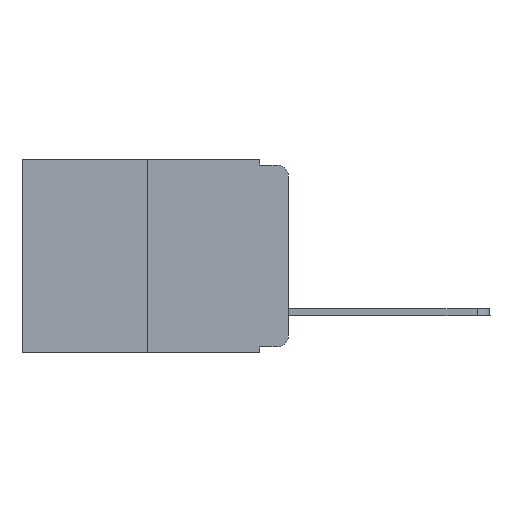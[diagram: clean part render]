
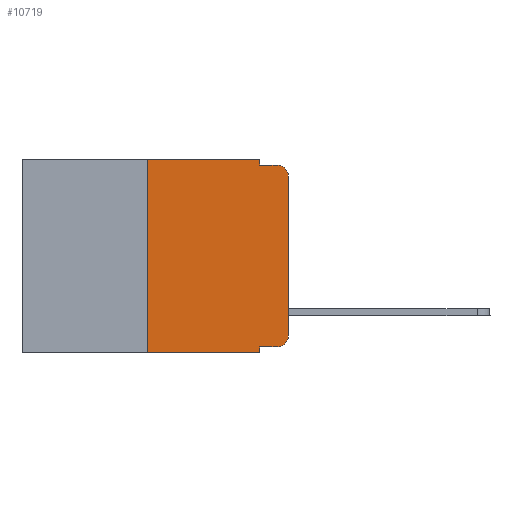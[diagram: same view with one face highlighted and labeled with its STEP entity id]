
A CAD part, left-side view. The second image highlights one B-rep face of the part: STEP entity #10719.
In plain terms, the highlighted planar face has unit normal (-1, 0, 0).
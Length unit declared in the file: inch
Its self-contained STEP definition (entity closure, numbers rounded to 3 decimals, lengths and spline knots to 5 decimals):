
#360 = CARTESIAN_POINT ( 'NONE',  ( 0., 0.051, -0.01 ) ) ;
#412 = VERTEX_POINT ( 'NONE', #360 ) ;
#806 = EDGE_CURVE ( 'NONE', #16024, #5300, #3020, .T. ) ;
#1102 = AXIS2_PLACEMENT_3D ( 'NONE', #13139, #18219, #8176 ) ;
#1482 = CARTESIAN_POINT ( 'NONE',  ( 0., 0.25, -0.343 ) ) ;
#1589 = DIRECTION ( 'NONE',  ( 0., 0., 1. ) ) ;
#2037 = DIRECTION ( 'NONE',  ( -1., 0., 0. ) ) ;
#2139 = CARTESIAN_POINT ( 'NONE',  ( 0., 0.051, -0.343 ) ) ;
#2553 = AXIS2_PLACEMENT_3D ( 'NONE', #12079, #2037, #7102 ) ;
#3020 = LINE ( 'NONE', #21550, #20329 ) ;
#3321 = VECTOR ( 'NONE', #19621, 39.37008 ) ;
#3622 = EDGE_CURVE ( 'NONE', #412, #6630, #21020, .T. ) ;
#3847 = ORIENTED_EDGE ( 'NONE', *, *, #3622, .F. ) ;
#4429 = LINE ( 'NONE', #4754, #17223 ) ;
#4602 = VECTOR ( 'NONE', #11974, 39.37008 ) ;
#4754 = CARTESIAN_POINT ( 'NONE',  ( 0., 0.473, -0.343 ) ) ;
#4831 = ORIENTED_EDGE ( 'NONE', *, *, #13532, .T. ) ;
#4868 = DIRECTION ( 'NONE',  ( 0., 0., -1. ) ) ;
#5271 = VECTOR ( 'NONE', #1589, 39.37008 ) ;
#5300 = VERTEX_POINT ( 'NONE', #2139 ) ;
#5643 = ORIENTED_EDGE ( 'NONE', *, *, #19200, .T. ) ;
#5779 = EDGE_CURVE ( 'NONE', #13026, #412, #11956, .T. ) ;
#5820 = VERTEX_POINT ( 'NONE', #17259 ) ;
#5857 = CARTESIAN_POINT ( 'NONE',  ( 0., 0.02, -0.333 ) ) ;
#5934 = DIRECTION ( 'NONE',  ( 0., -1., 0. ) ) ;
#6144 = VECTOR ( 'NONE', #17439, 39.37008 ) ;
#6237 = CARTESIAN_POINT ( 'NONE',  ( 0., 0.25, 0. ) ) ;
#6418 = CARTESIAN_POINT ( 'NONE',  ( 0., 0., -0.313 ) ) ;
#6488 = ORIENTED_EDGE ( 'NONE', *, *, #5779, .F. ) ;
#6512 = DIRECTION ( 'NONE',  ( 0., 0., -1. ) ) ;
#6630 = VERTEX_POINT ( 'NONE', #7505 ) ;
#7102 = DIRECTION ( 'NONE',  ( 0., 0., -1. ) ) ;
#7472 = EDGE_CURVE ( 'NONE', #21253, #19652, #8173, .T. ) ;
#7505 = CARTESIAN_POINT ( 'NONE',  ( 0., 0.02, -0.01 ) ) ;
#8173 = LINE ( 'NONE', #19317, #5271 ) ;
#8176 = DIRECTION ( 'NONE',  ( 0., 0., -1. ) ) ;
#9344 = EDGE_LOOP ( 'NONE', ( #11230, #16043, #3847, #6488, #15155, #11465, #5643, #19975, #10318, #4831 ) ) ;
#9807 = CIRCLE ( 'NONE', #2553, 0.02 ) ;
#9968 = EDGE_CURVE ( 'NONE', #19652, #13026, #12210, .T. ) ;
#10035 = DIRECTION ( 'NONE',  ( 1., 0., 0. ) ) ;
#10048 = LINE ( 'NONE', #17512, #6144 ) ;
#10067 = EDGE_CURVE ( 'NONE', #5820, #6630, #17485, .T. ) ;
#10318 = ORIENTED_EDGE ( 'NONE', *, *, #12422, .T. ) ;
#10517 = CARTESIAN_POINT ( 'NONE',  ( 0., 0.051, 0. ) ) ;
#10578 = LINE ( 'NONE', #13588, #4602 ) ;
#10644 = CARTESIAN_POINT ( 'NONE',  ( 0., 0.051, 0. ) ) ;
#10719 = ADVANCED_FACE ( 'NONE', ( #13483 ), #16716, .F. ) ;
#11230 = ORIENTED_EDGE ( 'NONE', *, *, #11560, .T. ) ;
#11465 = ORIENTED_EDGE ( 'NONE', *, *, #7472, .F. ) ;
#11560 = EDGE_CURVE ( 'NONE', #17374, #5820, #10048, .T. ) ;
#11956 = LINE ( 'NONE', #10517, #16962 ) ;
#11974 = DIRECTION ( 'NONE',  ( 0., -1., 0. ) ) ;
#12079 = CARTESIAN_POINT ( 'NONE',  ( 0., 0.02, -0.313 ) ) ;
#12210 = LINE ( 'NONE', #14386, #3321 ) ;
#12353 = CARTESIAN_POINT ( 'NONE',  ( 0., 0.051, -0.01 ) ) ;
#12422 = EDGE_CURVE ( 'NONE', #16024, #12492, #10578, .T. ) ;
#12492 = VERTEX_POINT ( 'NONE', #5857 ) ;
#13026 = VERTEX_POINT ( 'NONE', #10644 ) ;
#13139 = CARTESIAN_POINT ( 'NONE',  ( 0., 0.02, -0.03 ) ) ;
#13483 = FACE_OUTER_BOUND ( 'NONE', #9344, .T. ) ;
#13532 = EDGE_CURVE ( 'NONE', #12492, #17374, #9807, .T. ) ;
#13588 = CARTESIAN_POINT ( 'NONE',  ( 0., 0.051, -0.333 ) ) ;
#14386 = CARTESIAN_POINT ( 'NONE',  ( 0., 0.473, 0. ) ) ;
#15090 = CARTESIAN_POINT ( 'NONE',  ( 0., 0.473, 0. ) ) ;
#15155 = ORIENTED_EDGE ( 'NONE', *, *, #9968, .F. ) ;
#15705 = AXIS2_PLACEMENT_3D ( 'NONE', #15090, #10035, #4868 ) ;
#16024 = VERTEX_POINT ( 'NONE', #18580 ) ;
#16043 = ORIENTED_EDGE ( 'NONE', *, *, #10067, .T. ) ;
#16562 = VECTOR ( 'NONE', #5934, 39.37008 ) ;
#16716 = PLANE ( 'NONE',  #15705 ) ;
#16962 = VECTOR ( 'NONE', #17125, 39.37008 ) ;
#17125 = DIRECTION ( 'NONE',  ( 0., 0., -1. ) ) ;
#17223 = VECTOR ( 'NONE', #21526, 39.37008 ) ;
#17259 = CARTESIAN_POINT ( 'NONE',  ( 0., 0., -0.03 ) ) ;
#17374 = VERTEX_POINT ( 'NONE', #6418 ) ;
#17439 = DIRECTION ( 'NONE',  ( 0., 0., 1. ) ) ;
#17485 = CIRCLE ( 'NONE', #1102, 0.02 ) ;
#17512 = CARTESIAN_POINT ( 'NONE',  ( 0., 0., 0. ) ) ;
#18219 = DIRECTION ( 'NONE',  ( -1., 0., 0. ) ) ;
#18580 = CARTESIAN_POINT ( 'NONE',  ( 0., 0.051, -0.333 ) ) ;
#19200 = EDGE_CURVE ( 'NONE', #21253, #5300, #4429, .T. ) ;
#19317 = CARTESIAN_POINT ( 'NONE',  ( 0., 0.25, 0. ) ) ;
#19621 = DIRECTION ( 'NONE',  ( 0., -1., 0. ) ) ;
#19652 = VERTEX_POINT ( 'NONE', #6237 ) ;
#19975 = ORIENTED_EDGE ( 'NONE', *, *, #806, .F. ) ;
#20329 = VECTOR ( 'NONE', #6512, 39.37008 ) ;
#21020 = LINE ( 'NONE', #12353, #16562 ) ;
#21253 = VERTEX_POINT ( 'NONE', #1482 ) ;
#21526 = DIRECTION ( 'NONE',  ( 0., -1., 0. ) ) ;
#21550 = CARTESIAN_POINT ( 'NONE',  ( 0., 0.051, 0. ) ) ;
